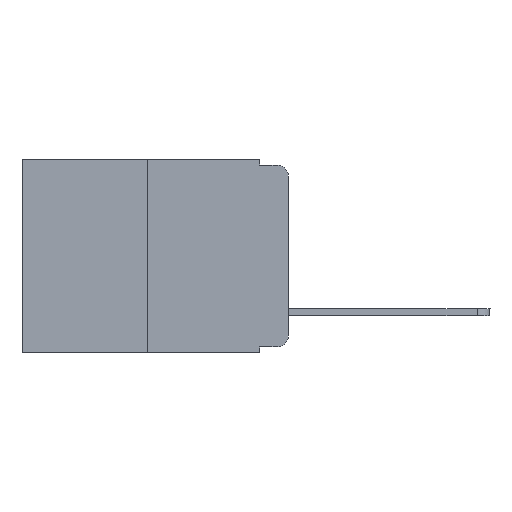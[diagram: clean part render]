
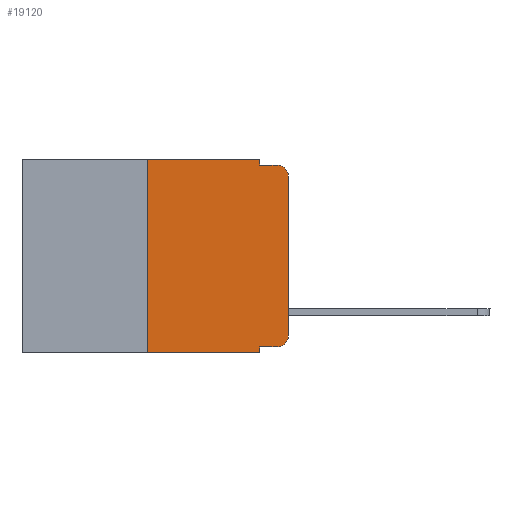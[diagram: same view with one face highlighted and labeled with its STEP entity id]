
A CAD part, left-side view. The second image highlights one B-rep face of the part: STEP entity #19120.
In plain terms, the highlighted planar face has unit normal (-1, 0, 0).
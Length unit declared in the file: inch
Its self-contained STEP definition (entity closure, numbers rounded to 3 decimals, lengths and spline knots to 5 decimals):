
#711 = LINE ( 'NONE', #5675, #7856 ) ;
#860 = DIRECTION ( 'NONE',  ( 0., 0., 1. ) ) ;
#1016 = DIRECTION ( 'NONE',  ( 0., -1., 0. ) ) ;
#1235 = VERTEX_POINT ( 'NONE', #7272 ) ;
#1491 = EDGE_CURVE ( 'NONE', #5561, #17564, #6728, .T. ) ;
#1540 = CARTESIAN_POINT ( 'NONE',  ( 0., 0.02, -0.313 ) ) ;
#1758 = ORIENTED_EDGE ( 'NONE', *, *, #18465, .T. ) ;
#1769 = CARTESIAN_POINT ( 'NONE',  ( 0., 0.051, 0. ) ) ;
#1793 = CARTESIAN_POINT ( 'NONE',  ( 0., 0.051, 0. ) ) ;
#1964 = CARTESIAN_POINT ( 'NONE',  ( 0., 0.25, 0. ) ) ;
#2053 = LINE ( 'NONE', #8600, #11477 ) ;
#2351 = DIRECTION ( 'NONE',  ( 1., 0., 0. ) ) ;
#2705 = EDGE_CURVE ( 'NONE', #5635, #18606, #16227, .T. ) ;
#2715 = EDGE_CURVE ( 'NONE', #1235, #13734, #17944, .T. ) ;
#3187 = LINE ( 'NONE', #11459, #19377 ) ;
#3207 = CARTESIAN_POINT ( 'NONE',  ( 0., 0.25, 0. ) ) ;
#3933 = CARTESIAN_POINT ( 'NONE',  ( 0., 0.051, -0.333 ) ) ;
#3960 = PLANE ( 'NONE',  #15279 ) ;
#4386 = DIRECTION ( 'NONE',  ( 0., -1., 0. ) ) ;
#4854 = EDGE_LOOP ( 'NONE', ( #13031, #17013, #17067, #9693, #19772, #9490, #1758, #19101, #15996, #8736 ) ) ;
#4961 = CIRCLE ( 'NONE', #20799, 0.02 ) ;
#5382 = EDGE_CURVE ( 'NONE', #16486, #5635, #3187, .T. ) ;
#5561 = VERTEX_POINT ( 'NONE', #3933 ) ;
#5635 = VERTEX_POINT ( 'NONE', #9084 ) ;
#5675 = CARTESIAN_POINT ( 'NONE',  ( 0., 0.051, -0.333 ) ) ;
#5859 = EDGE_CURVE ( 'NONE', #15779, #16062, #9056, .T. ) ;
#6219 = VECTOR ( 'NONE', #8547, 39.37008 ) ;
#6644 = DIRECTION ( 'NONE',  ( 0., -1., 0. ) ) ;
#6728 = LINE ( 'NONE', #1769, #6219 ) ;
#6859 = CARTESIAN_POINT ( 'NONE',  ( 0., 0.051, -0.01 ) ) ;
#7272 = CARTESIAN_POINT ( 'NONE',  ( 0., 0.25, -0.343 ) ) ;
#7448 = DIRECTION ( 'NONE',  ( 0., 0., -1. ) ) ;
#7551 = CARTESIAN_POINT ( 'NONE',  ( 0., 0.02, -0.03 ) ) ;
#7583 = CARTESIAN_POINT ( 'NONE',  ( 0., 0.473, -0.343 ) ) ;
#7853 = CARTESIAN_POINT ( 'NONE',  ( 0., 0., 0. ) ) ;
#7856 = VECTOR ( 'NONE', #4386, 39.37008 ) ;
#7897 = DIRECTION ( 'NONE',  ( 0., 0., -1. ) ) ;
#8051 = VECTOR ( 'NONE', #860, 39.37008 ) ;
#8539 = VERTEX_POINT ( 'NONE', #11700 ) ;
#8547 = DIRECTION ( 'NONE',  ( 0., 0., -1. ) ) ;
#8600 = CARTESIAN_POINT ( 'NONE',  ( 0., 0.473, 0. ) ) ;
#8736 = ORIENTED_EDGE ( 'NONE', *, *, #5859, .T. ) ;
#8894 = DIRECTION ( 'NONE',  ( 0., 0., -1. ) ) ;
#9056 = CIRCLE ( 'NONE', #13538, 0.02 ) ;
#9084 = CARTESIAN_POINT ( 'NONE',  ( 0., 0.051, -0.01 ) ) ;
#9490 = ORIENTED_EDGE ( 'NONE', *, *, #2715, .F. ) ;
#9507 = DIRECTION ( 'NONE',  ( -1., 0., 0. ) ) ;
#9693 = ORIENTED_EDGE ( 'NONE', *, *, #5382, .F. ) ;
#9758 = DIRECTION ( 'NONE',  ( 0., 0., 1. ) ) ;
#10187 = CARTESIAN_POINT ( 'NONE',  ( 0., 0.473, 0. ) ) ;
#11459 = CARTESIAN_POINT ( 'NONE',  ( 0., 0.051, 0. ) ) ;
#11477 = VECTOR ( 'NONE', #15170, 39.37008 ) ;
#11678 = EDGE_CURVE ( 'NONE', #5561, #15779, #711, .T. ) ;
#11700 = CARTESIAN_POINT ( 'NONE',  ( 0., 0., -0.03 ) ) ;
#12416 = LINE ( 'NONE', #7583, #18357 ) ;
#13031 = ORIENTED_EDGE ( 'NONE', *, *, #18793, .T. ) ;
#13538 = AXIS2_PLACEMENT_3D ( 'NONE', #1540, #9507, #7897 ) ;
#13557 = CARTESIAN_POINT ( 'NONE',  ( 0., 0., -0.313 ) ) ;
#13648 = FACE_OUTER_BOUND ( 'NONE', #4854, .T. ) ;
#13734 = VERTEX_POINT ( 'NONE', #1964 ) ;
#15170 = DIRECTION ( 'NONE',  ( 0., -1., 0. ) ) ;
#15279 = AXIS2_PLACEMENT_3D ( 'NONE', #10187, #2351, #8894 ) ;
#15779 = VERTEX_POINT ( 'NONE', #20699 ) ;
#15919 = CARTESIAN_POINT ( 'NONE',  ( 0., 0.051, -0.343 ) ) ;
#15996 = ORIENTED_EDGE ( 'NONE', *, *, #11678, .T. ) ;
#16062 = VERTEX_POINT ( 'NONE', #13557 ) ;
#16227 = LINE ( 'NONE', #6859, #20363 ) ;
#16486 = VERTEX_POINT ( 'NONE', #1793 ) ;
#17013 = ORIENTED_EDGE ( 'NONE', *, *, #17074, .T. ) ;
#17067 = ORIENTED_EDGE ( 'NONE', *, *, #2705, .F. ) ;
#17074 = EDGE_CURVE ( 'NONE', #8539, #18606, #4961, .T. ) ;
#17237 = DIRECTION ( 'NONE',  ( -1., 0., 0. ) ) ;
#17564 = VERTEX_POINT ( 'NONE', #15919 ) ;
#17613 = VECTOR ( 'NONE', #9758, 39.37008 ) ;
#17643 = LINE ( 'NONE', #7853, #8051 ) ;
#17722 = DIRECTION ( 'NONE',  ( 0., 0., -1. ) ) ;
#17944 = LINE ( 'NONE', #3207, #17613 ) ;
#18357 = VECTOR ( 'NONE', #1016, 39.37008 ) ;
#18465 = EDGE_CURVE ( 'NONE', #1235, #17564, #12416, .T. ) ;
#18606 = VERTEX_POINT ( 'NONE', #19823 ) ;
#18740 = EDGE_CURVE ( 'NONE', #13734, #16486, #2053, .T. ) ;
#18793 = EDGE_CURVE ( 'NONE', #16062, #8539, #17643, .T. ) ;
#19101 = ORIENTED_EDGE ( 'NONE', *, *, #1491, .F. ) ;
#19120 = ADVANCED_FACE ( 'NONE', ( #13648 ), #3960, .F. ) ;
#19377 = VECTOR ( 'NONE', #17722, 39.37008 ) ;
#19772 = ORIENTED_EDGE ( 'NONE', *, *, #18740, .F. ) ;
#19823 = CARTESIAN_POINT ( 'NONE',  ( 0., 0.02, -0.01 ) ) ;
#20363 = VECTOR ( 'NONE', #6644, 39.37008 ) ;
#20699 = CARTESIAN_POINT ( 'NONE',  ( 0., 0.02, -0.333 ) ) ;
#20799 = AXIS2_PLACEMENT_3D ( 'NONE', #7551, #17237, #7448 ) ;
